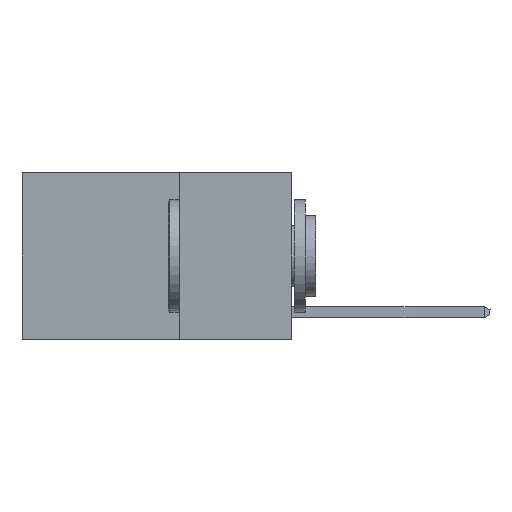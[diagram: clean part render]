
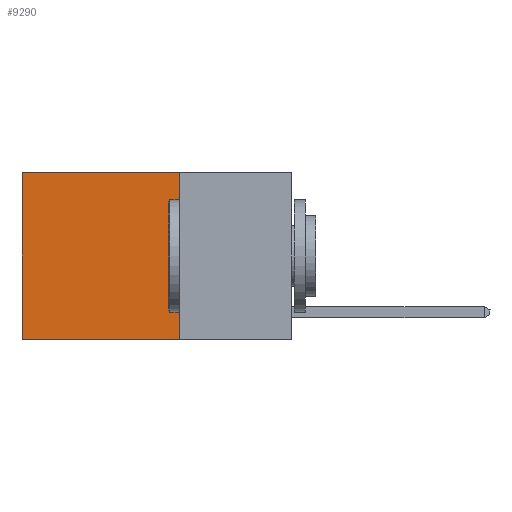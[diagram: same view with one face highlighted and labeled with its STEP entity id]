
A CAD part, left-side view. The second image highlights one B-rep face of the part: STEP entity #9290.
In plain terms, the highlighted planar face has unit normal (-1, 0, 0).
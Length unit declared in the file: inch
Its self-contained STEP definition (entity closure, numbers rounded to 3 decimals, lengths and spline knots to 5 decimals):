
#180 = ORIENTED_EDGE ( 'NONE', *, *, #9981, .F. ) ;
#508 = PLANE ( 'NONE',  #2148 ) ;
#876 = CARTESIAN_POINT ( 'NONE',  ( 0.2625, 0.25, -0.37 ) ) ;
#1407 = FACE_OUTER_BOUND ( 'NONE', #9874, .T. ) ;
#1623 = VECTOR ( 'NONE', #17156, 39.37008 ) ;
#2080 = DIRECTION ( 'NONE',  ( 0., 0., -1. ) ) ;
#2148 = AXIS2_PLACEMENT_3D ( 'NONE', #17448, #11375, #2080 ) ;
#2771 = DIRECTION ( 'NONE',  ( 0., 1., 0. ) ) ;
#3177 = VERTEX_POINT ( 'NONE', #19611 ) ;
#5268 = VERTEX_POINT ( 'NONE', #876 ) ;
#5424 = EDGE_CURVE ( 'NONE', #3177, #19578, #16889, .T. ) ;
#7244 = VECTOR ( 'NONE', #12663, 39.37008 ) ;
#7971 = CARTESIAN_POINT ( 'NONE',  ( 0.2625, 0.25, 0. ) ) ;
#8102 = EDGE_CURVE ( 'NONE', #19578, #15497, #17127, .T. ) ;
#8312 = ORIENTED_EDGE ( 'NONE', *, *, #5424, .T. ) ;
#8575 = ORIENTED_EDGE ( 'NONE', *, *, #17467, .F. ) ;
#9290 = ADVANCED_FACE ( 'NONE', ( #1407 ), #508, .F. ) ;
#9345 = ORIENTED_EDGE ( 'NONE', *, *, #8102, .T. ) ;
#9874 = EDGE_LOOP ( 'NONE', ( #9345, #8575, #180, #8312 ) ) ;
#9981 = EDGE_CURVE ( 'NONE', #3177, #5268, #13981, .T. ) ;
#11375 = DIRECTION ( 'NONE',  ( 1., 0., 0. ) ) ;
#11415 = DIRECTION ( 'NONE',  ( 0., 0., -1. ) ) ;
#11836 = LINE ( 'NONE', #15733, #7244 ) ;
#12663 = DIRECTION ( 'NONE',  ( 0., 1., 0. ) ) ;
#12856 = VECTOR ( 'NONE', #2771, 39.37008 ) ;
#13599 = CARTESIAN_POINT ( 'NONE',  ( 0.2625, 0.25, 0. ) ) ;
#13981 = LINE ( 'NONE', #7971, #1623 ) ;
#15497 = VERTEX_POINT ( 'NONE', #16819 ) ;
#15733 = CARTESIAN_POINT ( 'NONE',  ( 0.2625, 0.25, -0.37 ) ) ;
#16819 = CARTESIAN_POINT ( 'NONE',  ( 0.2625, 0.6, -0.37 ) ) ;
#16889 = LINE ( 'NONE', #13599, #12856 ) ;
#17127 = LINE ( 'NONE', #18997, #17603 ) ;
#17156 = DIRECTION ( 'NONE',  ( 0., 0., -1. ) ) ;
#17448 = CARTESIAN_POINT ( 'NONE',  ( 0.2625, 0.25, 0. ) ) ;
#17467 = EDGE_CURVE ( 'NONE', #5268, #15497, #11836, .T. ) ;
#17603 = VECTOR ( 'NONE', #11415, 39.37008 ) ;
#18997 = CARTESIAN_POINT ( 'NONE',  ( 0.2625, 0.6, 0. ) ) ;
#19397 = CARTESIAN_POINT ( 'NONE',  ( 0.2625, 0.6, 0. ) ) ;
#19578 = VERTEX_POINT ( 'NONE', #19397 ) ;
#19611 = CARTESIAN_POINT ( 'NONE',  ( 0.2625, 0.25, 0. ) ) ;
